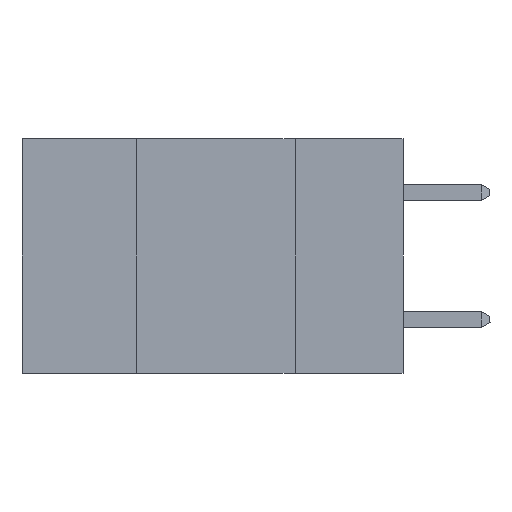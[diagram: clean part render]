
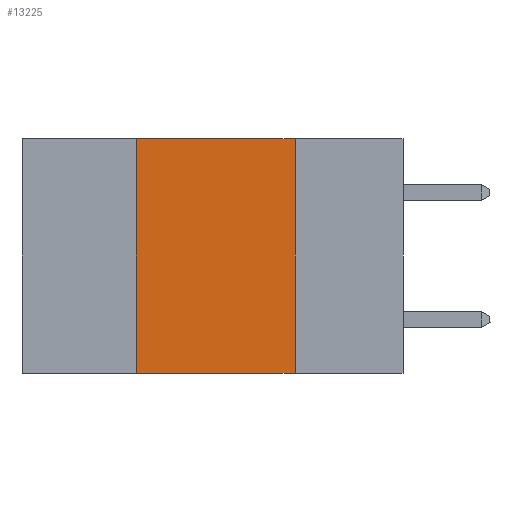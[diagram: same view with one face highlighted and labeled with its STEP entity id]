
A CAD part, left-side view. The second image highlights one B-rep face of the part: STEP entity #13225.
In plain terms, the highlighted planar face has unit normal (-1, 0, 0).
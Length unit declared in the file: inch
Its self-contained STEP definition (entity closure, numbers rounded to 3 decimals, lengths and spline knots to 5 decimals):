
#270 = CARTESIAN_POINT ( 'NONE',  ( 0., 0.17, 0. ) ) ;
#281 = ORIENTED_EDGE ( 'NONE', *, *, #9279, .T. ) ;
#596 = FACE_OUTER_BOUND ( 'NONE', #9922, .T. ) ;
#917 = EDGE_CURVE ( 'NONE', #2638, #6334, #12481, .T. ) ;
#939 = DIRECTION ( 'NONE',  ( 0., -1., 0. ) ) ;
#942 = VECTOR ( 'NONE', #939, 39.37008 ) ;
#1192 = EDGE_CURVE ( 'NONE', #9033, #2024, #3261, .T. ) ;
#1441 = PLANE ( 'NONE',  #6750 ) ;
#2024 = VERTEX_POINT ( 'NONE', #5626 ) ;
#2498 = CARTESIAN_POINT ( 'NONE',  ( 0., 0.6, 0. ) ) ;
#2544 = DIRECTION ( 'NONE',  ( 0., 0., -1. ) ) ;
#2638 = VERTEX_POINT ( 'NONE', #6678 ) ;
#3261 = LINE ( 'NONE', #13588, #6309 ) ;
#3265 = EDGE_CURVE ( 'NONE', #6334, #9033, #6984, .T. ) ;
#3976 = ORIENTED_EDGE ( 'NONE', *, *, #1192, .F. ) ;
#4554 = ORIENTED_EDGE ( 'NONE', *, *, #3265, .F. ) ;
#4912 = CARTESIAN_POINT ( 'NONE',  ( 0., 0.42, 0. ) ) ;
#5233 = DIRECTION ( 'NONE',  ( 0., -1., 0. ) ) ;
#5626 = CARTESIAN_POINT ( 'NONE',  ( 0., 0.17, -0.37 ) ) ;
#6309 = VECTOR ( 'NONE', #13424, 39.37008 ) ;
#6334 = VERTEX_POINT ( 'NONE', #4912 ) ;
#6678 = CARTESIAN_POINT ( 'NONE',  ( 0., 0.42, -0.37 ) ) ;
#6750 = AXIS2_PLACEMENT_3D ( 'NONE', #2498, #9302, #2544 ) ;
#6841 = LINE ( 'NONE', #11753, #9706 ) ;
#6984 = LINE ( 'NONE', #11909, #942 ) ;
#8436 = ORIENTED_EDGE ( 'NONE', *, *, #917, .F. ) ;
#9033 = VERTEX_POINT ( 'NONE', #270 ) ;
#9279 = EDGE_CURVE ( 'NONE', #2638, #2024, #6841, .T. ) ;
#9302 = DIRECTION ( 'NONE',  ( 1., 0., 0. ) ) ;
#9706 = VECTOR ( 'NONE', #5233, 39.37008 ) ;
#9922 = EDGE_LOOP ( 'NONE', ( #3976, #4554, #8436, #281 ) ) ;
#10079 = VECTOR ( 'NONE', #12163, 39.37008 ) ;
#11753 = CARTESIAN_POINT ( 'NONE',  ( 0., 0.6, -0.37 ) ) ;
#11909 = CARTESIAN_POINT ( 'NONE',  ( 0., 0.6, 0. ) ) ;
#12163 = DIRECTION ( 'NONE',  ( 0., 0., 1. ) ) ;
#12481 = LINE ( 'NONE', #13626, #10079 ) ;
#13225 = ADVANCED_FACE ( 'NONE', ( #596 ), #1441, .F. ) ;
#13424 = DIRECTION ( 'NONE',  ( 0., 0., -1. ) ) ;
#13588 = CARTESIAN_POINT ( 'NONE',  ( 0., 0.17, 0. ) ) ;
#13626 = CARTESIAN_POINT ( 'NONE',  ( 0., 0.42, 0. ) ) ;
